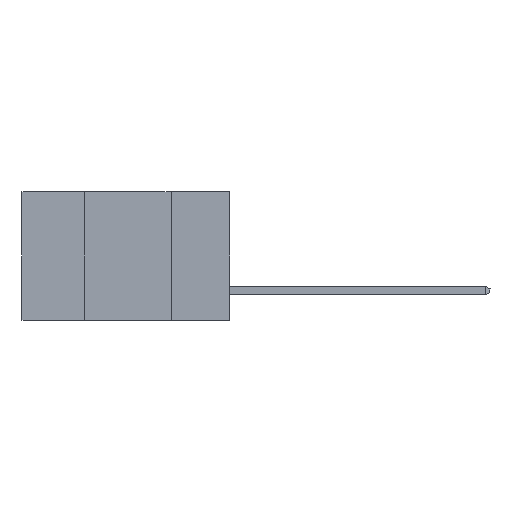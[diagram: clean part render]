
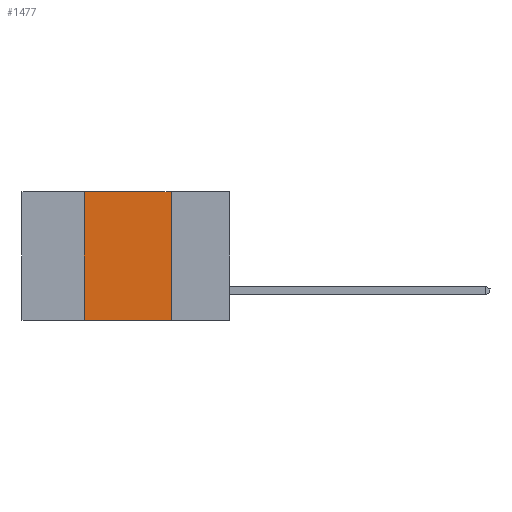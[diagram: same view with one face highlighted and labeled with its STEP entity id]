
A CAD part, left-side view. The second image highlights one B-rep face of the part: STEP entity #1477.
In plain terms, the highlighted planar face has unit normal (-1, 0, 0).
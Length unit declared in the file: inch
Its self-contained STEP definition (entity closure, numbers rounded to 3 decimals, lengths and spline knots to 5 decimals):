
#451 = PLANE ( 'NONE',  #512 ) ;
#512 = AXIS2_PLACEMENT_3D ( 'NONE', #4903, #2561, #1962 ) ;
#1395 = CARTESIAN_POINT ( 'NONE',  ( 0., 0.42, -0.37 ) ) ;
#1400 = LINE ( 'NONE', #5958, #3968 ) ;
#1477 = ADVANCED_FACE ( 'NONE', ( #9419 ), #451, .F. ) ;
#1572 = LINE ( 'NONE', #6746, #7077 ) ;
#1962 = DIRECTION ( 'NONE',  ( 0., 0., -1. ) ) ;
#2196 = CARTESIAN_POINT ( 'NONE',  ( 0., 0.17, -0.37 ) ) ;
#2311 = EDGE_CURVE ( 'NONE', #6165, #5059, #1400, .T. ) ;
#2561 = DIRECTION ( 'NONE',  ( 1., 0., 0. ) ) ;
#2768 = VECTOR ( 'NONE', #6849, 39.37008 ) ;
#2789 = ORIENTED_EDGE ( 'NONE', *, *, #8600, .F. ) ;
#2826 = EDGE_CURVE ( 'NONE', #6791, #3206, #1572, .T. ) ;
#3114 = LINE ( 'NONE', #9091, #7351 ) ;
#3168 = ORIENTED_EDGE ( 'NONE', *, *, #2311, .F. ) ;
#3206 = VERTEX_POINT ( 'NONE', #2196 ) ;
#3843 = DIRECTION ( 'NONE',  ( 0., -1., 0. ) ) ;
#3968 = VECTOR ( 'NONE', #3843, 39.37008 ) ;
#4792 = EDGE_LOOP ( 'NONE', ( #6645, #3168, #2789, #5261 ) ) ;
#4903 = CARTESIAN_POINT ( 'NONE',  ( 0., 0.6, 0. ) ) ;
#5059 = VERTEX_POINT ( 'NONE', #5398 ) ;
#5261 = ORIENTED_EDGE ( 'NONE', *, *, #2826, .T. ) ;
#5398 = CARTESIAN_POINT ( 'NONE',  ( 0., 0.17, 0. ) ) ;
#5958 = CARTESIAN_POINT ( 'NONE',  ( 0., 0.6, 0. ) ) ;
#6165 = VERTEX_POINT ( 'NONE', #9545 ) ;
#6645 = ORIENTED_EDGE ( 'NONE', *, *, #8226, .F. ) ;
#6746 = CARTESIAN_POINT ( 'NONE',  ( 0., 0.6, -0.37 ) ) ;
#6791 = VERTEX_POINT ( 'NONE', #1395 ) ;
#6849 = DIRECTION ( 'NONE',  ( 0., 0., 1. ) ) ;
#6898 = CARTESIAN_POINT ( 'NONE',  ( 0., 0.42, -0.37 ) ) ;
#7077 = VECTOR ( 'NONE', #8322, 39.37008 ) ;
#7351 = VECTOR ( 'NONE', #8434, 39.37008 ) ;
#8226 = EDGE_CURVE ( 'NONE', #5059, #3206, #3114, .T. ) ;
#8322 = DIRECTION ( 'NONE',  ( 0., -1., 0. ) ) ;
#8434 = DIRECTION ( 'NONE',  ( 0., 0., -1. ) ) ;
#8600 = EDGE_CURVE ( 'NONE', #6791, #6165, #9079, .T. ) ;
#9079 = LINE ( 'NONE', #6898, #2768 ) ;
#9091 = CARTESIAN_POINT ( 'NONE',  ( 0., 0.17, -0.37 ) ) ;
#9419 = FACE_OUTER_BOUND ( 'NONE', #4792, .T. ) ;
#9545 = CARTESIAN_POINT ( 'NONE',  ( 0., 0.42, 0. ) ) ;
